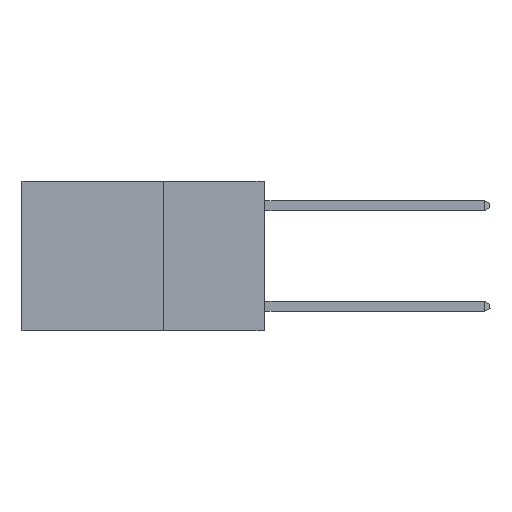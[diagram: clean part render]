
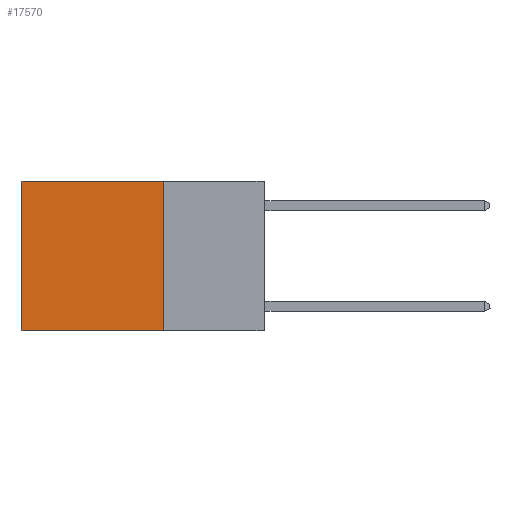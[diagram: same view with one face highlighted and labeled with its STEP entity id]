
A CAD part, left-side view. The second image highlights one B-rep face of the part: STEP entity #17570.
In plain terms, the highlighted planar face has unit normal (-1, 0, 0).
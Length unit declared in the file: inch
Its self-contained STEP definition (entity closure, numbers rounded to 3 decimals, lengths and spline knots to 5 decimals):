
#378 = LINE ( 'NONE', #18900, #5222 ) ;
#1592 = VECTOR ( 'NONE', #12362, 39.37008 ) ;
#1911 = CARTESIAN_POINT ( 'NONE',  ( 0.2625, 0.25, 0. ) ) ;
#3324 = EDGE_LOOP ( 'NONE', ( #7369, #15777, #9989, #20858 ) ) ;
#3599 = LINE ( 'NONE', #3719, #1592 ) ;
#3605 = LINE ( 'NONE', #1911, #18752 ) ;
#3719 = CARTESIAN_POINT ( 'NONE',  ( 0.2625, 0.25, 0. ) ) ;
#4001 = VERTEX_POINT ( 'NONE', #6713 ) ;
#5216 = CARTESIAN_POINT ( 'NONE',  ( 0.2625, 0.6, 0. ) ) ;
#5222 = VECTOR ( 'NONE', #14941, 39.37008 ) ;
#6713 = CARTESIAN_POINT ( 'NONE',  ( 0.2625, 0.25, 0. ) ) ;
#7369 = ORIENTED_EDGE ( 'NONE', *, *, #10068, .T. ) ;
#8063 = EDGE_CURVE ( 'NONE', #4001, #9680, #3599, .T. ) ;
#9327 = EDGE_CURVE ( 'NONE', #4001, #24617, #3605, .T. ) ;
#9555 = LINE ( 'NONE', #17928, #25346 ) ;
#9680 = VERTEX_POINT ( 'NONE', #5216 ) ;
#9973 = PLANE ( 'NONE',  #18598 ) ;
#9989 = ORIENTED_EDGE ( 'NONE', *, *, #9327, .F. ) ;
#10068 = EDGE_CURVE ( 'NONE', #9680, #17890, #378, .T. ) ;
#10114 = CARTESIAN_POINT ( 'NONE',  ( 0.2625, 0.25, 0. ) ) ;
#10361 = DIRECTION ( 'NONE',  ( 0., 0., -1. ) ) ;
#12362 = DIRECTION ( 'NONE',  ( 0., 1., 0. ) ) ;
#14941 = DIRECTION ( 'NONE',  ( 0., 0., -1. ) ) ;
#15777 = ORIENTED_EDGE ( 'NONE', *, *, #22388, .F. ) ;
#16174 = CARTESIAN_POINT ( 'NONE',  ( 0.2625, 0.25, -0.37 ) ) ;
#17570 = ADVANCED_FACE ( 'NONE', ( #26136 ), #9973, .F. ) ;
#17890 = VERTEX_POINT ( 'NONE', #24074 ) ;
#17928 = CARTESIAN_POINT ( 'NONE',  ( 0.2625, 0.25, -0.37 ) ) ;
#18598 = AXIS2_PLACEMENT_3D ( 'NONE', #10114, #20774, #10361 ) ;
#18752 = VECTOR ( 'NONE', #20449, 39.37008 ) ;
#18900 = CARTESIAN_POINT ( 'NONE',  ( 0.2625, 0.6, 0. ) ) ;
#20449 = DIRECTION ( 'NONE',  ( 0., 0., -1. ) ) ;
#20774 = DIRECTION ( 'NONE',  ( 1., 0., 0. ) ) ;
#20858 = ORIENTED_EDGE ( 'NONE', *, *, #8063, .T. ) ;
#22166 = DIRECTION ( 'NONE',  ( 0., 1., 0. ) ) ;
#22388 = EDGE_CURVE ( 'NONE', #24617, #17890, #9555, .T. ) ;
#24074 = CARTESIAN_POINT ( 'NONE',  ( 0.2625, 0.6, -0.37 ) ) ;
#24617 = VERTEX_POINT ( 'NONE', #16174 ) ;
#25346 = VECTOR ( 'NONE', #22166, 39.37008 ) ;
#26136 = FACE_OUTER_BOUND ( 'NONE', #3324, .T. ) ;
